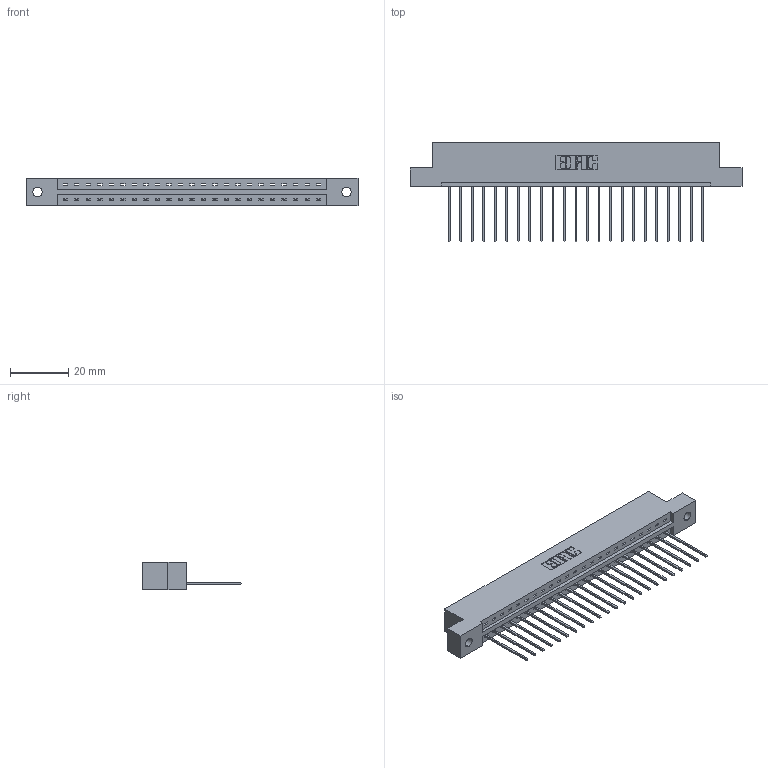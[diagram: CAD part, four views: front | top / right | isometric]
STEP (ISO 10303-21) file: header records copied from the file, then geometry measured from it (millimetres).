
FILE_DESCRIPTION (( 'STEP AP203' ), '1' );
FILE_NAME ('387-023-541-102.STEP', '2018-09-14T08:12:29', ( '' ), ( '' ), 'SwSTEP 2.0', 'SolidWorks 2016', '' );
FILE_SCHEMA (( 'CONFIG_CONTROL_DESIGN' ));
Length unit declared in the file: inch
Products named in the file (3): 337 Part_Flush Mounting Lugs - 0.128 Dia; 345-292-001_345-293-141; 387-023-541-102
Assembly tree (24 placements, depth 2):
  387-023-541-102
    337 Part_Flush Mounting Lugs - 0.128 Dia
    345-292-001_345-293-141  x23
Bounding box: 114.15 x 34.3 x 9.4 mm (x, y, z)
Volume: 11665.2 mm3; surface area: 12145.8 mm2
Topology: 24 solids, 24 shells, 1540 faces, 4635 edges, 3058 vertices
Faces by surface type: plane 1128, cylinder 412
Entity records: 19575 total; most frequent: CARTESIAN_POINT 3415, ORIENTED_EDGE 3374, DIRECTION 2913, EDGE_CURVE 1687, VECTOR 1559, LINE 1559, VERTEX_POINT 1122, AXIS2_PLACEMENT_3D 677
